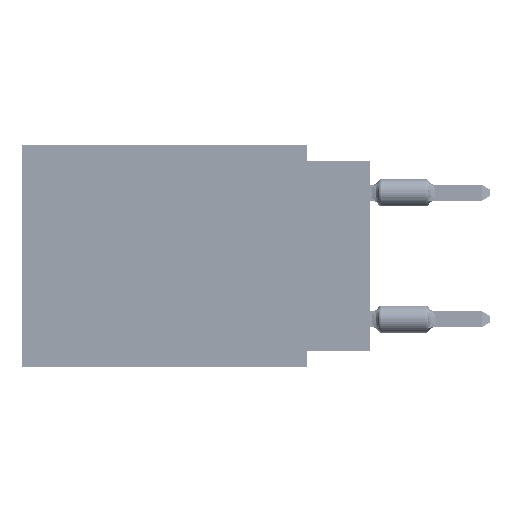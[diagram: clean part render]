
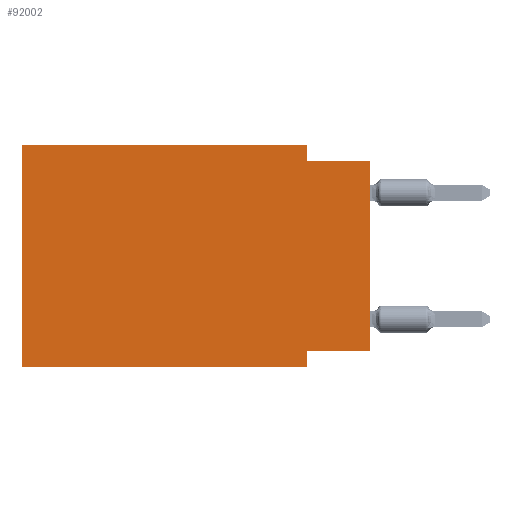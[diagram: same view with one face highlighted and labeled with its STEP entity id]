
A CAD part, left-side view. The second image highlights one B-rep face of the part: STEP entity #92002.
In plain terms, the highlighted planar face has unit normal (-1, 0, 0).
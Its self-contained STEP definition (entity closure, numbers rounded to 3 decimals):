
#3883 = VERTEX_POINT ( 'NONE', #10533 ) ;
#10533 = CARTESIAN_POINT ( 'NONE',  ( 0., 2.54, 0. ) ) ;
#11203 = DIRECTION ( 'NONE',  ( 0., 1., 0. ) ) ;
#12510 = VECTOR ( 'NONE', #47898, 1000. ) ;
#15119 = LINE ( 'NONE', #87672, #100205 ) ;
#15987 = VERTEX_POINT ( 'NONE', #30219 ) ;
#16176 = EDGE_CURVE ( 'NONE', #15987, #35139, #40229, .T. ) ;
#21001 = LINE ( 'NONE', #45339, #49469 ) ;
#21846 = EDGE_CURVE ( 'NONE', #60070, #39886, #66517, .T. ) ;
#22398 = VECTOR ( 'NONE', #24915, 1000. ) ;
#24137 = DIRECTION ( 'NONE',  ( 0., 0., -1. ) ) ;
#24915 = DIRECTION ( 'NONE',  ( 0., -1., 0. ) ) ;
#25376 = EDGE_CURVE ( 'NONE', #47328, #80154, #83753, .T. ) ;
#26295 = DIRECTION ( 'NONE',  ( 0., 0., 1. ) ) ;
#27332 = CARTESIAN_POINT ( 'NONE',  ( 0., 13.97, 0. ) ) ;
#27533 = CARTESIAN_POINT ( 'NONE',  ( 0., 13.97, -8.89 ) ) ;
#28675 = CARTESIAN_POINT ( 'NONE',  ( 0., 0., -8.255 ) ) ;
#29984 = DIRECTION ( 'NONE',  ( 0., -1., 0. ) ) ;
#30219 = CARTESIAN_POINT ( 'NONE',  ( 0., 2.54, -0.635 ) ) ;
#35139 = VERTEX_POINT ( 'NONE', #91572 ) ;
#36318 = VECTOR ( 'NONE', #11203, 1000. ) ;
#37275 = DIRECTION ( 'NONE',  ( 0., 0., -1. ) ) ;
#38831 = CARTESIAN_POINT ( 'NONE',  ( 0., 2.54, -8.89 ) ) ;
#39886 = VERTEX_POINT ( 'NONE', #95022 ) ;
#40229 = LINE ( 'NONE', #72531, #22398 ) ;
#40279 = ORIENTED_EDGE ( 'NONE', *, *, #65196, .F. ) ;
#44484 = ORIENTED_EDGE ( 'NONE', *, *, #21846, .F. ) ;
#45339 = CARTESIAN_POINT ( 'NONE',  ( 0., 13.97, -8.89 ) ) ;
#47142 = CARTESIAN_POINT ( 'NONE',  ( 0., 2.54, -8.89 ) ) ;
#47328 = VERTEX_POINT ( 'NONE', #56063 ) ;
#47898 = DIRECTION ( 'NONE',  ( 0., -1., 0. ) ) ;
#48786 = AXIS2_PLACEMENT_3D ( 'NONE', #60751, #100992, #24137 ) ;
#49375 = VECTOR ( 'NONE', #26295, 1000. ) ;
#49469 = VECTOR ( 'NONE', #29984, 1000. ) ;
#49682 = ORIENTED_EDGE ( 'NONE', *, *, #25376, .F. ) ;
#53942 = LINE ( 'NONE', #54979, #82781 ) ;
#54979 = CARTESIAN_POINT ( 'NONE',  ( 0., 2.54, 0. ) ) ;
#55871 = DIRECTION ( 'NONE',  ( 0., 0., 1. ) ) ;
#56063 = CARTESIAN_POINT ( 'NONE',  ( 0., 0., -8.255 ) ) ;
#57198 = ORIENTED_EDGE ( 'NONE', *, *, #102032, .T. ) ;
#60070 = VERTEX_POINT ( 'NONE', #27533 ) ;
#60751 = CARTESIAN_POINT ( 'NONE',  ( 0., 13.97, 0. ) ) ;
#61269 = EDGE_LOOP ( 'NONE', ( #57198, #94915, #40279, #100198, #44484, #66400, #72092, #49682 ) ) ;
#65196 = EDGE_CURVE ( 'NONE', #3883, #15987, #53942, .T. ) ;
#66043 = CARTESIAN_POINT ( 'NONE',  ( 0., 2.54, -8.255 ) ) ;
#66400 = ORIENTED_EDGE ( 'NONE', *, *, #85651, .T. ) ;
#66517 = LINE ( 'NONE', #27332, #49375 ) ;
#68701 = PLANE ( 'NONE',  #48786 ) ;
#69475 = EDGE_CURVE ( 'NONE', #80154, #88729, #78031, .T. ) ;
#70175 = LINE ( 'NONE', #104560, #12510 ) ;
#72092 = ORIENTED_EDGE ( 'NONE', *, *, #69475, .F. ) ;
#72531 = CARTESIAN_POINT ( 'NONE',  ( 0., 0., -0.635 ) ) ;
#76412 = VECTOR ( 'NONE', #37275, 1000. ) ;
#78031 = LINE ( 'NONE', #38831, #76412 ) ;
#78729 = EDGE_CURVE ( 'NONE', #39886, #3883, #70175, .T. ) ;
#80154 = VERTEX_POINT ( 'NONE', #66043 ) ;
#82781 = VECTOR ( 'NONE', #85229, 1000. ) ;
#83753 = LINE ( 'NONE', #28675, #36318 ) ;
#85229 = DIRECTION ( 'NONE',  ( 0., 0., -1. ) ) ;
#85651 = EDGE_CURVE ( 'NONE', #60070, #88729, #21001, .T. ) ;
#87672 = CARTESIAN_POINT ( 'NONE',  ( 0., 0., 0. ) ) ;
#88729 = VERTEX_POINT ( 'NONE', #47142 ) ;
#91572 = CARTESIAN_POINT ( 'NONE',  ( 0., 0., -0.635 ) ) ;
#92002 = ADVANCED_FACE ( 'NONE', ( #102017 ), #68701, .F. ) ;
#94915 = ORIENTED_EDGE ( 'NONE', *, *, #16176, .F. ) ;
#95022 = CARTESIAN_POINT ( 'NONE',  ( 0., 13.97, 0. ) ) ;
#100198 = ORIENTED_EDGE ( 'NONE', *, *, #78729, .F. ) ;
#100205 = VECTOR ( 'NONE', #55871, 1000. ) ;
#100992 = DIRECTION ( 'NONE',  ( 1., 0., 0. ) ) ;
#102017 = FACE_OUTER_BOUND ( 'NONE', #61269, .T. ) ;
#102032 = EDGE_CURVE ( 'NONE', #47328, #35139, #15119, .T. ) ;
#104560 = CARTESIAN_POINT ( 'NONE',  ( 0., 13.97, 0. ) ) ;
